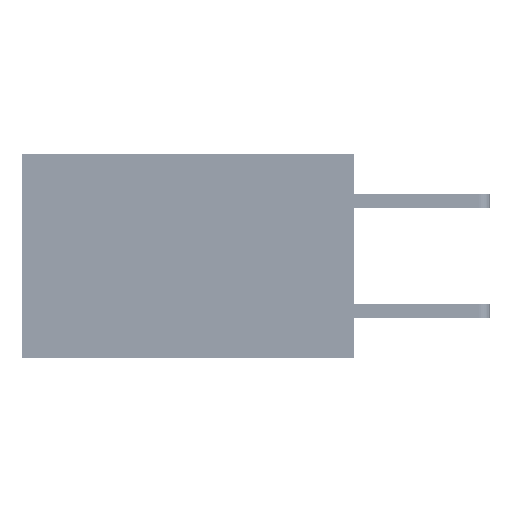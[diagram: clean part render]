
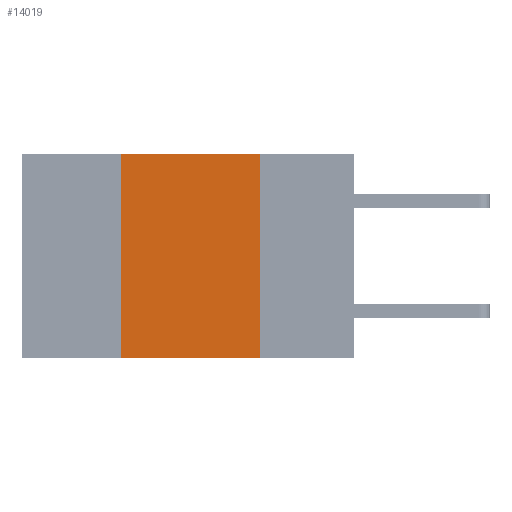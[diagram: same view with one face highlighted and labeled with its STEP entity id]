
A CAD part, left-side view. The second image highlights one B-rep face of the part: STEP entity #14019.
In plain terms, the highlighted planar face has unit normal (-1, 0, 0).
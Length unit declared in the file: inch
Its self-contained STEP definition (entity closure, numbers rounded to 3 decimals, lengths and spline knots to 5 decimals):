
#831 = DIRECTION ( 'NONE',  ( 0., 0., -1. ) ) ;
#930 = VERTEX_POINT ( 'NONE', #21554 ) ;
#1305 = ORIENTED_EDGE ( 'NONE', *, *, #15726, .T. ) ;
#4121 = FACE_OUTER_BOUND ( 'NONE', #46620, .T. ) ;
#5171 = EDGE_CURVE ( 'NONE', #28585, #930, #32006, .T. ) ;
#6416 = LINE ( 'NONE', #9466, #35464 ) ;
#6669 = DIRECTION ( 'NONE',  ( 0., -1., 0. ) ) ;
#6888 = VERTEX_POINT ( 'NONE', #31487 ) ;
#9466 = CARTESIAN_POINT ( 'NONE',  ( 0., 0.6, -0.37 ) ) ;
#9916 = CARTESIAN_POINT ( 'NONE',  ( 0., 0.6, 0. ) ) ;
#13587 = CARTESIAN_POINT ( 'NONE',  ( 0., 0.42, 0. ) ) ;
#14019 = ADVANCED_FACE ( 'NONE', ( #4121 ), #30656, .F. ) ;
#14346 = VERTEX_POINT ( 'NONE', #29859 ) ;
#15695 = DIRECTION ( 'NONE',  ( 1., 0., 0. ) ) ;
#15722 = EDGE_CURVE ( 'NONE', #14346, #6888, #28296, .T. ) ;
#15726 = EDGE_CURVE ( 'NONE', #14346, #930, #6416, .T. ) ;
#17406 = DIRECTION ( 'NONE',  ( 0., 0., 1. ) ) ;
#20611 = VECTOR ( 'NONE', #17406, 39.37008 ) ;
#21554 = CARTESIAN_POINT ( 'NONE',  ( 0., 0.17, -0.37 ) ) ;
#22015 = EDGE_CURVE ( 'NONE', #6888, #28585, #32650, .T. ) ;
#25824 = AXIS2_PLACEMENT_3D ( 'NONE', #27464, #15695, #831 ) ;
#27464 = CARTESIAN_POINT ( 'NONE',  ( 0., 0.6, 0. ) ) ;
#28296 = LINE ( 'NONE', #13587, #20611 ) ;
#28585 = VERTEX_POINT ( 'NONE', #35156 ) ;
#29859 = CARTESIAN_POINT ( 'NONE',  ( 0., 0.42, -0.37 ) ) ;
#30656 = PLANE ( 'NONE',  #25824 ) ;
#31487 = CARTESIAN_POINT ( 'NONE',  ( 0., 0.42, 0. ) ) ;
#32006 = LINE ( 'NONE', #39834, #44581 ) ;
#32650 = LINE ( 'NONE', #9916, #47548 ) ;
#35156 = CARTESIAN_POINT ( 'NONE',  ( 0., 0.17, 0. ) ) ;
#35464 = VECTOR ( 'NONE', #6669, 39.37008 ) ;
#38268 = ORIENTED_EDGE ( 'NONE', *, *, #15722, .F. ) ;
#39834 = CARTESIAN_POINT ( 'NONE',  ( 0., 0.17, 0. ) ) ;
#41443 = ORIENTED_EDGE ( 'NONE', *, *, #22015, .F. ) ;
#44173 = DIRECTION ( 'NONE',  ( 0., -1., 0. ) ) ;
#44208 = ORIENTED_EDGE ( 'NONE', *, *, #5171, .F. ) ;
#44581 = VECTOR ( 'NONE', #47159, 39.37008 ) ;
#46620 = EDGE_LOOP ( 'NONE', ( #44208, #41443, #38268, #1305 ) ) ;
#47159 = DIRECTION ( 'NONE',  ( 0., 0., -1. ) ) ;
#47548 = VECTOR ( 'NONE', #44173, 39.37008 ) ;
